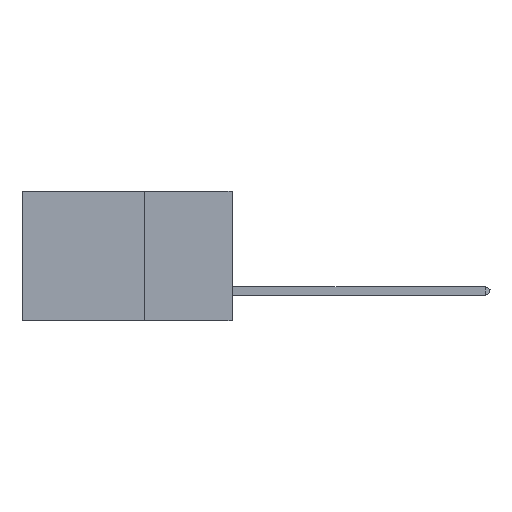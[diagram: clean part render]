
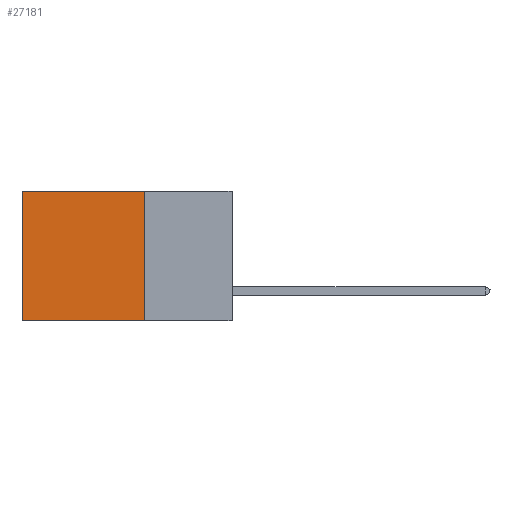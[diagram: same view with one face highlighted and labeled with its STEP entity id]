
A CAD part, left-side view. The second image highlights one B-rep face of the part: STEP entity #27181.
In plain terms, the highlighted planar face has unit normal (-1, 0, 0).
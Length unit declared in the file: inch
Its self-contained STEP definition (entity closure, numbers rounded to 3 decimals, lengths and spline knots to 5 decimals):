
#34 = EDGE_CURVE ( 'NONE', #13160, #15709, #33098, .T. ) ;
#625 = VECTOR ( 'NONE', #12760, 39.37008 ) ;
#1617 = PLANE ( 'NONE',  #9084 ) ;
#2289 = VECTOR ( 'NONE', #31375, 39.37008 ) ;
#3012 = LINE ( 'NONE', #24676, #16058 ) ;
#3965 = CARTESIAN_POINT ( 'NONE',  ( 0.2875, 0.25, 0. ) ) ;
#4245 = VECTOR ( 'NONE', #17646, 39.37008 ) ;
#7424 = ORIENTED_EDGE ( 'NONE', *, *, #34, .F. ) ;
#7446 = CARTESIAN_POINT ( 'NONE',  ( 0.2875, 0.25, 0. ) ) ;
#7651 = CARTESIAN_POINT ( 'NONE',  ( 0.2875, 0.25, 0. ) ) ;
#9084 = AXIS2_PLACEMENT_3D ( 'NONE', #7446, #10228, #21030 ) ;
#9628 = LINE ( 'NONE', #9694, #2289 ) ;
#9694 = CARTESIAN_POINT ( 'NONE',  ( 0.2875, 0.25, 0. ) ) ;
#10228 = DIRECTION ( 'NONE',  ( 1., 0., 0. ) ) ;
#10330 = CARTESIAN_POINT ( 'NONE',  ( 0.2875, 0.25, -0.37 ) ) ;
#10622 = VERTEX_POINT ( 'NONE', #23229 ) ;
#12760 = DIRECTION ( 'NONE',  ( 0., 1., 0. ) ) ;
#13094 = EDGE_CURVE ( 'NONE', #26408, #13160, #9628, .T. ) ;
#13105 = CARTESIAN_POINT ( 'NONE',  ( 0.2875, 0.25, -0.37 ) ) ;
#13160 = VERTEX_POINT ( 'NONE', #13105 ) ;
#14013 = FACE_OUTER_BOUND ( 'NONE', #26314, .T. ) ;
#14765 = EDGE_CURVE ( 'NONE', #10622, #15709, #3012, .T. ) ;
#15709 = VERTEX_POINT ( 'NONE', #23226 ) ;
#16058 = VECTOR ( 'NONE', #27417, 39.37008 ) ;
#16200 = ORIENTED_EDGE ( 'NONE', *, *, #14765, .T. ) ;
#17646 = DIRECTION ( 'NONE',  ( 0., 1., 0. ) ) ;
#20878 = EDGE_CURVE ( 'NONE', #26408, #10622, #30146, .T. ) ;
#21030 = DIRECTION ( 'NONE',  ( 0., 0., -1. ) ) ;
#23226 = CARTESIAN_POINT ( 'NONE',  ( 0.2875, 0.6, -0.37 ) ) ;
#23229 = CARTESIAN_POINT ( 'NONE',  ( 0.2875, 0.6, 0. ) ) ;
#24676 = CARTESIAN_POINT ( 'NONE',  ( 0.2875, 0.6, 0. ) ) ;
#26314 = EDGE_LOOP ( 'NONE', ( #16200, #7424, #34348, #33999 ) ) ;
#26408 = VERTEX_POINT ( 'NONE', #7651 ) ;
#27181 = ADVANCED_FACE ( 'NONE', ( #14013 ), #1617, .F. ) ;
#27417 = DIRECTION ( 'NONE',  ( 0., 0., -1. ) ) ;
#30146 = LINE ( 'NONE', #3965, #4245 ) ;
#31375 = DIRECTION ( 'NONE',  ( 0., 0., -1. ) ) ;
#33098 = LINE ( 'NONE', #10330, #625 ) ;
#33999 = ORIENTED_EDGE ( 'NONE', *, *, #20878, .T. ) ;
#34348 = ORIENTED_EDGE ( 'NONE', *, *, #13094, .F. ) ;
